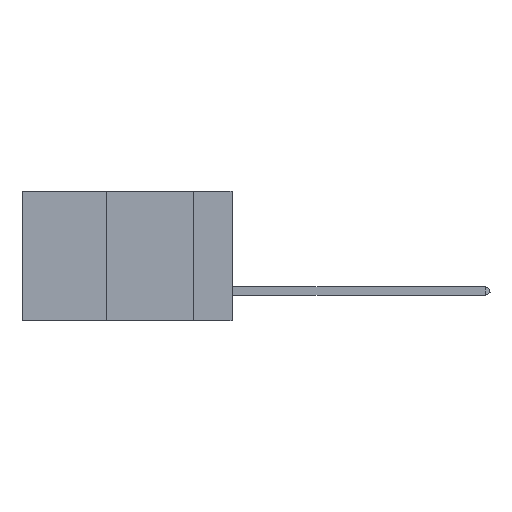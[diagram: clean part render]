
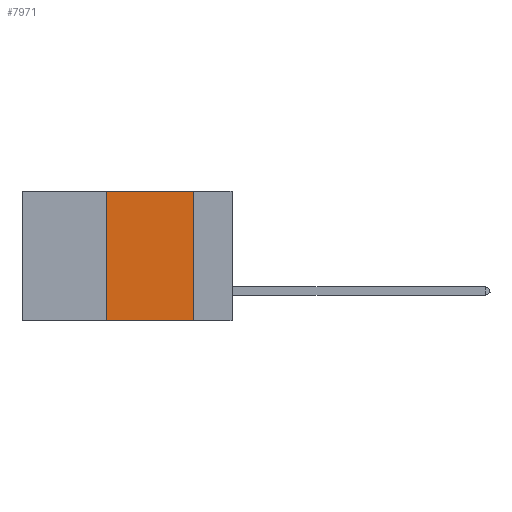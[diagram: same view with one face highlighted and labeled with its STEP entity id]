
A CAD part, left-side view. The second image highlights one B-rep face of the part: STEP entity #7971.
In plain terms, the highlighted planar face has unit normal (-1, 0, 0).
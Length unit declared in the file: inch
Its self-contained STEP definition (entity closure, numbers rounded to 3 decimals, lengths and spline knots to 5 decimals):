
#76 = ORIENTED_EDGE ( 'NONE', *, *, #7121, .F. ) ;
#414 = AXIS2_PLACEMENT_3D ( 'NONE', #9555, #1157, #1268 ) ;
#650 = VERTEX_POINT ( 'NONE', #6337 ) ;
#1157 = DIRECTION ( 'NONE',  ( 1., 0., 0. ) ) ;
#1268 = DIRECTION ( 'NONE',  ( 0., 0., -1. ) ) ;
#1543 = ORIENTED_EDGE ( 'NONE', *, *, #10012, .T. ) ;
#2602 = VERTEX_POINT ( 'NONE', #8497 ) ;
#2731 = VERTEX_POINT ( 'NONE', #7390 ) ;
#2816 = CARTESIAN_POINT ( 'NONE',  ( 0., 0.36, -0.37 ) ) ;
#3074 = VECTOR ( 'NONE', #9000, 39.37008 ) ;
#3220 = CARTESIAN_POINT ( 'NONE',  ( 0., 0.11, 0. ) ) ;
#3803 = VECTOR ( 'NONE', #7113, 39.37008 ) ;
#3915 = LINE ( 'NONE', #8209, #7027 ) ;
#4038 = VECTOR ( 'NONE', #8741, 39.37008 ) ;
#4065 = LINE ( 'NONE', #10498, #3803 ) ;
#4358 = EDGE_CURVE ( 'NONE', #4676, #650, #6376, .T. ) ;
#4676 = VERTEX_POINT ( 'NONE', #2816 ) ;
#5061 = DIRECTION ( 'NONE',  ( 0., -1., 0. ) ) ;
#5528 = LINE ( 'NONE', #3220, #3074 ) ;
#6337 = CARTESIAN_POINT ( 'NONE',  ( 0., 0.36, 0. ) ) ;
#6376 = LINE ( 'NONE', #8716, #4038 ) ;
#6864 = ORIENTED_EDGE ( 'NONE', *, *, #9277, .F. ) ;
#7027 = VECTOR ( 'NONE', #5061, 39.37008 ) ;
#7113 = DIRECTION ( 'NONE',  ( 0., -1., 0. ) ) ;
#7121 = EDGE_CURVE ( 'NONE', #2602, #2731, #5528, .T. ) ;
#7390 = CARTESIAN_POINT ( 'NONE',  ( 0., 0.11, -0.37 ) ) ;
#7810 = EDGE_LOOP ( 'NONE', ( #76, #6864, #9798, #1543 ) ) ;
#7971 = ADVANCED_FACE ( 'NONE', ( #10588 ), #8581, .F. ) ;
#8209 = CARTESIAN_POINT ( 'NONE',  ( 0., 0.6, -0.37 ) ) ;
#8497 = CARTESIAN_POINT ( 'NONE',  ( 0., 0.11, 0. ) ) ;
#8581 = PLANE ( 'NONE',  #414 ) ;
#8716 = CARTESIAN_POINT ( 'NONE',  ( 0., 0.36, 0. ) ) ;
#8741 = DIRECTION ( 'NONE',  ( 0., 0., 1. ) ) ;
#9000 = DIRECTION ( 'NONE',  ( 0., 0., -1. ) ) ;
#9277 = EDGE_CURVE ( 'NONE', #650, #2602, #4065, .T. ) ;
#9555 = CARTESIAN_POINT ( 'NONE',  ( 0., 0.6, 0. ) ) ;
#9798 = ORIENTED_EDGE ( 'NONE', *, *, #4358, .F. ) ;
#10012 = EDGE_CURVE ( 'NONE', #4676, #2731, #3915, .T. ) ;
#10498 = CARTESIAN_POINT ( 'NONE',  ( 0., 0.6, 0. ) ) ;
#10588 = FACE_OUTER_BOUND ( 'NONE', #7810, .T. ) ;
